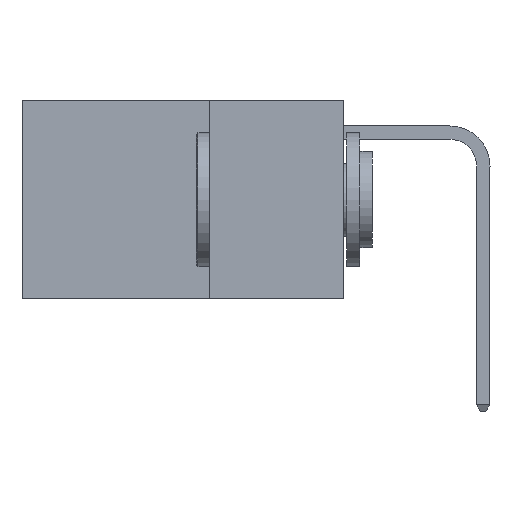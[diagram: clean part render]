
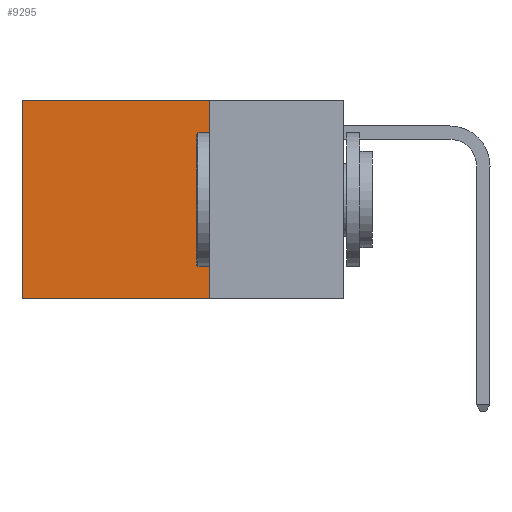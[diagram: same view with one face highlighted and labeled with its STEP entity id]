
A CAD part, left-side view. The second image highlights one B-rep face of the part: STEP entity #9295.
In plain terms, the highlighted planar face has unit normal (-1, 0, 0).
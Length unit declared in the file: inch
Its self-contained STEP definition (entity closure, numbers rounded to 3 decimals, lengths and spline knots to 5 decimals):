
#34 = VERTEX_POINT ( 'NONE', #11595 ) ;
#594 = DIRECTION ( 'NONE',  ( 0., 1., 0. ) ) ;
#632 = FACE_OUTER_BOUND ( 'NONE', #22871, .T. ) ;
#1549 = VECTOR ( 'NONE', #594, 39.37008 ) ;
#1688 = CARTESIAN_POINT ( 'NONE',  ( 0.2625, 0.25, 0. ) ) ;
#2465 = DIRECTION ( 'NONE',  ( 0., 0., -1. ) ) ;
#2735 = ORIENTED_EDGE ( 'NONE', *, *, #13592, .T. ) ;
#3677 = PLANE ( 'NONE',  #15476 ) ;
#5124 = ORIENTED_EDGE ( 'NONE', *, *, #13328, .F. ) ;
#5626 = EDGE_CURVE ( 'NONE', #34, #7666, #9146, .T. ) ;
#6093 = LINE ( 'NONE', #21142, #15822 ) ;
#6818 = LINE ( 'NONE', #14321, #1549 ) ;
#7015 = VECTOR ( 'NONE', #18349, 39.37008 ) ;
#7666 = VERTEX_POINT ( 'NONE', #21833 ) ;
#8550 = CARTESIAN_POINT ( 'NONE',  ( 0.2625, 0.25, 0. ) ) ;
#9146 = LINE ( 'NONE', #12333, #13692 ) ;
#9295 = ADVANCED_FACE ( 'NONE', ( #632 ), #3677, .F. ) ;
#9334 = ORIENTED_EDGE ( 'NONE', *, *, #5626, .T. ) ;
#9591 = DIRECTION ( 'NONE',  ( 0., 0., -1. ) ) ;
#11595 = CARTESIAN_POINT ( 'NONE',  ( 0.2625, 0.6, 0. ) ) ;
#12277 = CARTESIAN_POINT ( 'NONE',  ( 0.2625, 0.25, 0. ) ) ;
#12333 = CARTESIAN_POINT ( 'NONE',  ( 0.2625, 0.6, 0. ) ) ;
#12802 = LINE ( 'NONE', #8550, #7015 ) ;
#13328 = EDGE_CURVE ( 'NONE', #19579, #18491, #12802, .T. ) ;
#13592 = EDGE_CURVE ( 'NONE', #19579, #34, #6093, .T. ) ;
#13692 = VECTOR ( 'NONE', #2465, 39.37008 ) ;
#14321 = CARTESIAN_POINT ( 'NONE',  ( 0.2625, 0.25, -0.37 ) ) ;
#15476 = AXIS2_PLACEMENT_3D ( 'NONE', #1688, #21271, #9591 ) ;
#15822 = VECTOR ( 'NONE', #19202, 39.37008 ) ;
#18349 = DIRECTION ( 'NONE',  ( 0., 0., -1. ) ) ;
#18491 = VERTEX_POINT ( 'NONE', #24444 ) ;
#19042 = EDGE_CURVE ( 'NONE', #18491, #7666, #6818, .T. ) ;
#19202 = DIRECTION ( 'NONE',  ( 0., 1., 0. ) ) ;
#19579 = VERTEX_POINT ( 'NONE', #12277 ) ;
#21142 = CARTESIAN_POINT ( 'NONE',  ( 0.2625, 0.25, 0. ) ) ;
#21271 = DIRECTION ( 'NONE',  ( 1., 0., 0. ) ) ;
#21833 = CARTESIAN_POINT ( 'NONE',  ( 0.2625, 0.6, -0.37 ) ) ;
#22871 = EDGE_LOOP ( 'NONE', ( #9334, #22957, #5124, #2735 ) ) ;
#22957 = ORIENTED_EDGE ( 'NONE', *, *, #19042, .F. ) ;
#24444 = CARTESIAN_POINT ( 'NONE',  ( 0.2625, 0.25, -0.37 ) ) ;
